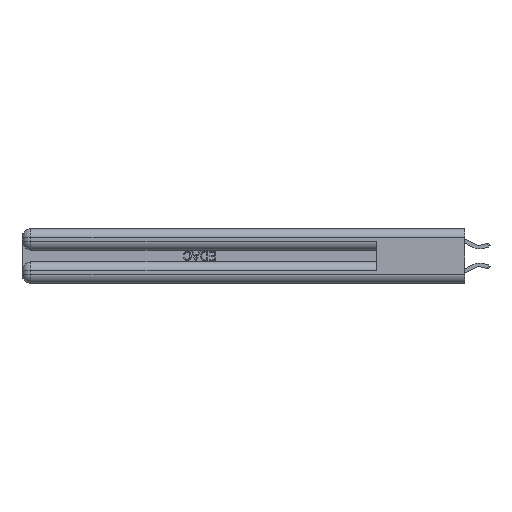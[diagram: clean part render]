
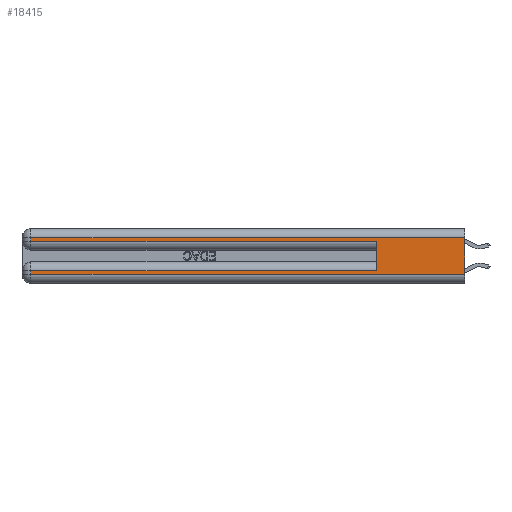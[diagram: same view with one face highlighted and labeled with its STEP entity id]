
A CAD part, left-side view. The second image highlights one B-rep face of the part: STEP entity #18415.
In plain terms, the highlighted planar face has unit normal (-1, 0, 0).
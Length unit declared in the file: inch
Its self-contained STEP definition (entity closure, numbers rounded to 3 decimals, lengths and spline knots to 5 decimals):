
#163 = DIRECTION ( 'NONE',  ( 0., 1., 0. ) ) ;
#1420 = DIRECTION ( 'NONE',  ( 0., 0., 1. ) ) ;
#2292 = ORIENTED_EDGE ( 'NONE', *, *, #19852, .T. ) ;
#2324 = VECTOR ( 'NONE', #12809, 39.37008 ) ;
#2543 = CARTESIAN_POINT ( 'NONE',  ( 0., 0., 0.37 ) ) ;
#2583 = CARTESIAN_POINT ( 'NONE',  ( 0., 0.6, 0.285 ) ) ;
#2856 = LINE ( 'NONE', #24965, #12813 ) ;
#3002 = CARTESIAN_POINT ( 'NONE',  ( 0., 0., 0.31 ) ) ;
#3171 = LINE ( 'NONE', #2543, #12554 ) ;
#3811 = VERTEX_POINT ( 'NONE', #2583 ) ;
#3876 = CARTESIAN_POINT ( 'NONE',  ( 0., 2.94, 0.285 ) ) ;
#5283 = VERTEX_POINT ( 'NONE', #27851 ) ;
#5539 = DIRECTION ( 'NONE',  ( 0., 0., -1. ) ) ;
#5899 = DIRECTION ( 'NONE',  ( 0., 0., -1. ) ) ;
#5965 = EDGE_CURVE ( 'NONE', #29563, #17950, #21496, .T. ) ;
#6679 = EDGE_CURVE ( 'NONE', #14966, #5283, #3171, .T. ) ;
#6946 = VERTEX_POINT ( 'NONE', #22520 ) ;
#7909 = CARTESIAN_POINT ( 'NONE',  ( 0., 0., 0.285 ) ) ;
#8561 = CARTESIAN_POINT ( 'NONE',  ( 0., 0., 0.06 ) ) ;
#9107 = ORIENTED_EDGE ( 'NONE', *, *, #5965, .T. ) ;
#9112 = CARTESIAN_POINT ( 'NONE',  ( 0., 2.94, 0.31 ) ) ;
#9554 = CARTESIAN_POINT ( 'NONE',  ( 0., 0.6, 0.085 ) ) ;
#10973 = PLANE ( 'NONE',  #18451 ) ;
#11707 = EDGE_CURVE ( 'NONE', #15096, #6946, #12656, .T. ) ;
#11861 = VERTEX_POINT ( 'NONE', #27334 ) ;
#12554 = VECTOR ( 'NONE', #5539, 39.37008 ) ;
#12656 = LINE ( 'NONE', #29077, #27841 ) ;
#12809 = DIRECTION ( 'NONE',  ( 0., 1., 0. ) ) ;
#12813 = VECTOR ( 'NONE', #29080, 39.37008 ) ;
#13035 = EDGE_LOOP ( 'NONE', ( #21671, #15155, #9107, #27034, #13878, #15007, #14749, #2292 ) ) ;
#13162 = DIRECTION ( 'NONE',  ( 0., -1., 0. ) ) ;
#13878 = ORIENTED_EDGE ( 'NONE', *, *, #21915, .F. ) ;
#14749 = ORIENTED_EDGE ( 'NONE', *, *, #15756, .T. ) ;
#14966 = VERTEX_POINT ( 'NONE', #30226 ) ;
#15007 = ORIENTED_EDGE ( 'NONE', *, *, #11707, .T. ) ;
#15096 = VERTEX_POINT ( 'NONE', #9554 ) ;
#15155 = ORIENTED_EDGE ( 'NONE', *, *, #18953, .T. ) ;
#15172 = DIRECTION ( 'NONE',  ( 0., -1., 0. ) ) ;
#15267 = DIRECTION ( 'NONE',  ( 0., 0., -1. ) ) ;
#15380 = DIRECTION ( 'NONE',  ( 1., 0., 0. ) ) ;
#15756 = EDGE_CURVE ( 'NONE', #6946, #11861, #2856, .T. ) ;
#15799 = EDGE_CURVE ( 'NONE', #17950, #3811, #27032, .T. ) ;
#17950 = VERTEX_POINT ( 'NONE', #3876 ) ;
#18415 = ADVANCED_FACE ( 'NONE', ( #27391 ), #10973, .F. ) ;
#18451 = AXIS2_PLACEMENT_3D ( 'NONE', #27545, #15380, #5899 ) ;
#18953 = EDGE_CURVE ( 'NONE', #14966, #29563, #24646, .T. ) ;
#19846 = VECTOR ( 'NONE', #15172, 39.37008 ) ;
#19852 = EDGE_CURVE ( 'NONE', #11861, #5283, #30195, .T. ) ;
#21011 = CARTESIAN_POINT ( 'NONE',  ( 0., 0.6, 0.145 ) ) ;
#21496 = LINE ( 'NONE', #21655, #27562 ) ;
#21655 = CARTESIAN_POINT ( 'NONE',  ( 0., 2.94, 0.37 ) ) ;
#21671 = ORIENTED_EDGE ( 'NONE', *, *, #6679, .F. ) ;
#21915 = EDGE_CURVE ( 'NONE', #15096, #3811, #30941, .T. ) ;
#22520 = CARTESIAN_POINT ( 'NONE',  ( 0., 2.94, 0.085 ) ) ;
#24646 = LINE ( 'NONE', #3002, #2324 ) ;
#24965 = CARTESIAN_POINT ( 'NONE',  ( 0., 2.94, 0.37 ) ) ;
#25018 = VECTOR ( 'NONE', #13162, 39.37008 ) ;
#26602 = VECTOR ( 'NONE', #1420, 39.37008 ) ;
#27032 = LINE ( 'NONE', #7909, #19846 ) ;
#27034 = ORIENTED_EDGE ( 'NONE', *, *, #15799, .T. ) ;
#27334 = CARTESIAN_POINT ( 'NONE',  ( 0., 2.94, 0.06 ) ) ;
#27391 = FACE_OUTER_BOUND ( 'NONE', #13035, .T. ) ;
#27545 = CARTESIAN_POINT ( 'NONE',  ( 0., 0., 0.37 ) ) ;
#27562 = VECTOR ( 'NONE', #15267, 39.37008 ) ;
#27841 = VECTOR ( 'NONE', #163, 39.37008 ) ;
#27851 = CARTESIAN_POINT ( 'NONE',  ( 0., 0., 0.06 ) ) ;
#29077 = CARTESIAN_POINT ( 'NONE',  ( 0., 0., 0.085 ) ) ;
#29080 = DIRECTION ( 'NONE',  ( 0., 0., -1. ) ) ;
#29563 = VERTEX_POINT ( 'NONE', #9112 ) ;
#30195 = LINE ( 'NONE', #8561, #25018 ) ;
#30226 = CARTESIAN_POINT ( 'NONE',  ( 0., 0., 0.31 ) ) ;
#30941 = LINE ( 'NONE', #21011, #26602 ) ;
